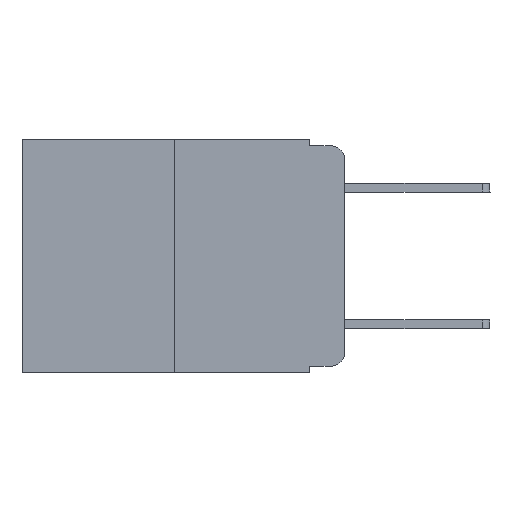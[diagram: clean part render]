
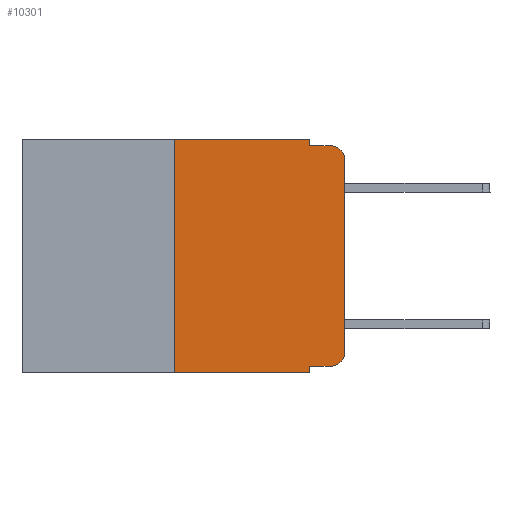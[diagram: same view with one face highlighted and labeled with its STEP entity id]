
A CAD part, left-side view. The second image highlights one B-rep face of the part: STEP entity #10301.
In plain terms, the highlighted planar face has unit normal (-1, 0, 0).
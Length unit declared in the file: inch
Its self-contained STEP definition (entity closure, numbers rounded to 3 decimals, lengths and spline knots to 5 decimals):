
#17 = VECTOR ( 'NONE', #6620, 39.37008 ) ;
#170 = DIRECTION ( 'NONE',  ( 0., -1., 0. ) ) ;
#559 = PLANE ( 'NONE',  #2240 ) ;
#714 = VERTEX_POINT ( 'NONE', #8445 ) ;
#879 = CARTESIAN_POINT ( 'NONE',  ( 0., 0.051, -0.343 ) ) ;
#929 = CARTESIAN_POINT ( 'NONE',  ( 0., 0.02, -0.01 ) ) ;
#947 = ORIENTED_EDGE ( 'NONE', *, *, #4354, .F. ) ;
#1363 = DIRECTION ( 'NONE',  ( 0., 0., -1. ) ) ;
#1400 = DIRECTION ( 'NONE',  ( -1., 0., 0. ) ) ;
#1704 = CARTESIAN_POINT ( 'NONE',  ( 0., 0., -0.03 ) ) ;
#1828 = CARTESIAN_POINT ( 'NONE',  ( 0., 0.051, 0. ) ) ;
#1830 = EDGE_CURVE ( 'NONE', #2435, #4646, #10079, .T. ) ;
#1860 = DIRECTION ( 'NONE',  ( 0., 0., -1. ) ) ;
#2240 = AXIS2_PLACEMENT_3D ( 'NONE', #10792, #4825, #5740 ) ;
#2435 = VERTEX_POINT ( 'NONE', #9808 ) ;
#2647 = VERTEX_POINT ( 'NONE', #929 ) ;
#3032 = LINE ( 'NONE', #1828, #8204 ) ;
#3074 = VERTEX_POINT ( 'NONE', #3088 ) ;
#3088 = CARTESIAN_POINT ( 'NONE',  ( 0., 0.02, -0.333 ) ) ;
#3141 = CARTESIAN_POINT ( 'NONE',  ( 0., 0.051, -0.333 ) ) ;
#3143 = ORIENTED_EDGE ( 'NONE', *, *, #6963, .F. ) ;
#3313 = VERTEX_POINT ( 'NONE', #879 ) ;
#3734 = LINE ( 'NONE', #6850, #9657 ) ;
#3809 = EDGE_LOOP ( 'NONE', ( #7889, #7315, #6472, #8081, #947, #3143, #7557, #9871, #6505, #8243 ) ) ;
#3811 = FACE_OUTER_BOUND ( 'NONE', #3809, .T. ) ;
#3822 = VERTEX_POINT ( 'NONE', #1704 ) ;
#3922 = EDGE_CURVE ( 'NONE', #6293, #3074, #10458, .T. ) ;
#3984 = CARTESIAN_POINT ( 'NONE',  ( 0., 0.02, -0.313 ) ) ;
#4284 = DIRECTION ( 'NONE',  ( 0., 0., 1. ) ) ;
#4354 = EDGE_CURVE ( 'NONE', #5124, #2435, #7075, .T. ) ;
#4490 = LINE ( 'NONE', #7592, #10935 ) ;
#4519 = EDGE_CURVE ( 'NONE', #714, #3313, #3734, .T. ) ;
#4526 = EDGE_CURVE ( 'NONE', #8782, #3822, #9414, .T. ) ;
#4646 = VERTEX_POINT ( 'NONE', #6305 ) ;
#4740 = CARTESIAN_POINT ( 'NONE',  ( 0., 0.051, 0. ) ) ;
#4825 = DIRECTION ( 'NONE',  ( 1., 0., 0. ) ) ;
#5124 = VERTEX_POINT ( 'NONE', #8454 ) ;
#5516 = LINE ( 'NONE', #5830, #10657 ) ;
#5740 = DIRECTION ( 'NONE',  ( 0., 0., -1. ) ) ;
#5830 = CARTESIAN_POINT ( 'NONE',  ( 0., 0.051, -0.01 ) ) ;
#5899 = CARTESIAN_POINT ( 'NONE',  ( 0., 0., 0. ) ) ;
#6293 = VERTEX_POINT ( 'NONE', #3141 ) ;
#6305 = CARTESIAN_POINT ( 'NONE',  ( 0., 0.051, -0.01 ) ) ;
#6410 = VECTOR ( 'NONE', #8867, 39.37008 ) ;
#6472 = ORIENTED_EDGE ( 'NONE', *, *, #6475, .F. ) ;
#6475 = EDGE_CURVE ( 'NONE', #4646, #2647, #5516, .T. ) ;
#6505 = ORIENTED_EDGE ( 'NONE', *, *, #3922, .T. ) ;
#6620 = DIRECTION ( 'NONE',  ( 0., -1., 0. ) ) ;
#6654 = EDGE_CURVE ( 'NONE', #6293, #3313, #3032, .T. ) ;
#6850 = CARTESIAN_POINT ( 'NONE',  ( 0., 0.473, -0.343 ) ) ;
#6963 = EDGE_CURVE ( 'NONE', #714, #5124, #4490, .T. ) ;
#7075 = LINE ( 'NONE', #9972, #17 ) ;
#7146 = DIRECTION ( 'NONE',  ( -1., 0., 0. ) ) ;
#7315 = ORIENTED_EDGE ( 'NONE', *, *, #8700, .T. ) ;
#7557 = ORIENTED_EDGE ( 'NONE', *, *, #4519, .T. ) ;
#7592 = CARTESIAN_POINT ( 'NONE',  ( 0., 0.25, 0. ) ) ;
#7702 = DIRECTION ( 'NONE',  ( 0., -1., 0. ) ) ;
#7716 = CARTESIAN_POINT ( 'NONE',  ( 0., 0.051, -0.333 ) ) ;
#7889 = ORIENTED_EDGE ( 'NONE', *, *, #4526, .T. ) ;
#7986 = AXIS2_PLACEMENT_3D ( 'NONE', #3984, #1400, #1363 ) ;
#8081 = ORIENTED_EDGE ( 'NONE', *, *, #1830, .F. ) ;
#8204 = VECTOR ( 'NONE', #9413, 39.37008 ) ;
#8243 = ORIENTED_EDGE ( 'NONE', *, *, #10249, .T. ) ;
#8315 = CIRCLE ( 'NONE', #7986, 0.02 ) ;
#8445 = CARTESIAN_POINT ( 'NONE',  ( 0., 0.25, -0.343 ) ) ;
#8454 = CARTESIAN_POINT ( 'NONE',  ( 0., 0.25, 0. ) ) ;
#8509 = VECTOR ( 'NONE', #10165, 39.37008 ) ;
#8551 = CIRCLE ( 'NONE', #10648, 0.02 ) ;
#8574 = CARTESIAN_POINT ( 'NONE',  ( 0., 0.02, -0.03 ) ) ;
#8644 = CARTESIAN_POINT ( 'NONE',  ( 0., 0., -0.313 ) ) ;
#8700 = EDGE_CURVE ( 'NONE', #3822, #2647, #8551, .T. ) ;
#8782 = VERTEX_POINT ( 'NONE', #8644 ) ;
#8867 = DIRECTION ( 'NONE',  ( 0., 0., -1. ) ) ;
#9413 = DIRECTION ( 'NONE',  ( 0., 0., -1. ) ) ;
#9414 = LINE ( 'NONE', #5899, #8509 ) ;
#9418 = VECTOR ( 'NONE', #170, 39.37008 ) ;
#9657 = VECTOR ( 'NONE', #7702, 39.37008 ) ;
#9808 = CARTESIAN_POINT ( 'NONE',  ( 0., 0.051, 0. ) ) ;
#9871 = ORIENTED_EDGE ( 'NONE', *, *, #6654, .F. ) ;
#9972 = CARTESIAN_POINT ( 'NONE',  ( 0., 0.473, 0. ) ) ;
#10079 = LINE ( 'NONE', #4740, #6410 ) ;
#10165 = DIRECTION ( 'NONE',  ( 0., 0., 1. ) ) ;
#10249 = EDGE_CURVE ( 'NONE', #3074, #8782, #8315, .T. ) ;
#10301 = ADVANCED_FACE ( 'NONE', ( #3811 ), #559, .F. ) ;
#10458 = LINE ( 'NONE', #7716, #9418 ) ;
#10648 = AXIS2_PLACEMENT_3D ( 'NONE', #8574, #7146, #1860 ) ;
#10657 = VECTOR ( 'NONE', #10946, 39.37008 ) ;
#10792 = CARTESIAN_POINT ( 'NONE',  ( 0., 0.473, 0. ) ) ;
#10935 = VECTOR ( 'NONE', #4284, 39.37008 ) ;
#10946 = DIRECTION ( 'NONE',  ( 0., -1., 0. ) ) ;
